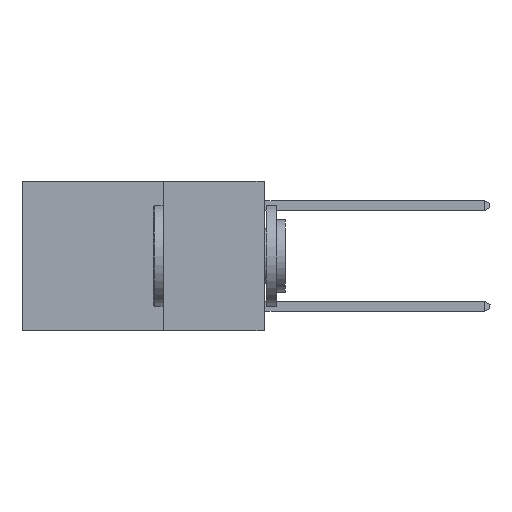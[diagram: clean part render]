
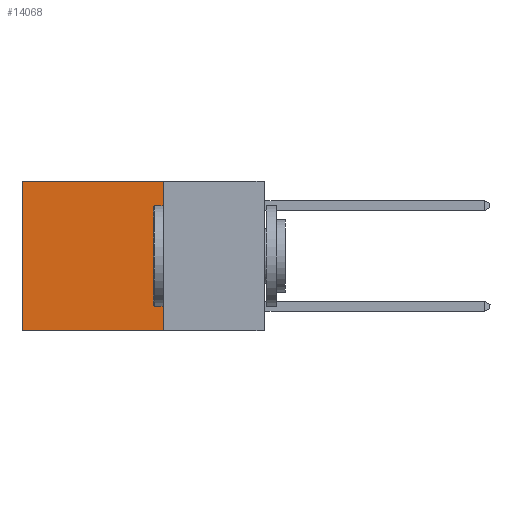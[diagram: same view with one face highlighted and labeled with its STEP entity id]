
A CAD part, left-side view. The second image highlights one B-rep face of the part: STEP entity #14068.
In plain terms, the highlighted planar face has unit normal (-1, 0, 0).
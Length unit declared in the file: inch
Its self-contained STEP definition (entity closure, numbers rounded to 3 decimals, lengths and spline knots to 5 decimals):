
#286 = CARTESIAN_POINT ( 'NONE',  ( 0.2625, 0.25, 0. ) ) ;
#1740 = AXIS2_PLACEMENT_3D ( 'NONE', #13962, #5261, #15449 ) ;
#1745 = EDGE_LOOP ( 'NONE', ( #13700, #10122, #11207, #15705 ) ) ;
#2292 = DIRECTION ( 'NONE',  ( 0., 0., -1. ) ) ;
#3195 = EDGE_CURVE ( 'NONE', #9516, #5290, #6839, .T. ) ;
#3809 = PLANE ( 'NONE',  #1740 ) ;
#4184 = EDGE_CURVE ( 'NONE', #5290, #18615, #13611, .T. ) ;
#5187 = EDGE_CURVE ( 'NONE', #9516, #7630, #16520, .T. ) ;
#5261 = DIRECTION ( 'NONE',  ( 1., 0., 0. ) ) ;
#5290 = VERTEX_POINT ( 'NONE', #10677 ) ;
#6839 = LINE ( 'NONE', #17581, #14090 ) ;
#7414 = DIRECTION ( 'NONE',  ( 0., 1., 0. ) ) ;
#7630 = VERTEX_POINT ( 'NONE', #16922 ) ;
#7952 = DIRECTION ( 'NONE',  ( 0., 1., 0. ) ) ;
#8009 = CARTESIAN_POINT ( 'NONE',  ( 0.2625, 0.25, 0. ) ) ;
#8986 = DIRECTION ( 'NONE',  ( 0., 0., -1. ) ) ;
#9244 = VECTOR ( 'NONE', #8986, 39.37008 ) ;
#9344 = CARTESIAN_POINT ( 'NONE',  ( 0.2625, 0.25, -0.37 ) ) ;
#9516 = VERTEX_POINT ( 'NONE', #8009 ) ;
#9976 = FACE_OUTER_BOUND ( 'NONE', #1745, .T. ) ;
#10122 = ORIENTED_EDGE ( 'NONE', *, *, #11447, .F. ) ;
#10677 = CARTESIAN_POINT ( 'NONE',  ( 0.2625, 0.6, 0. ) ) ;
#11207 = ORIENTED_EDGE ( 'NONE', *, *, #5187, .F. ) ;
#11447 = EDGE_CURVE ( 'NONE', #7630, #18615, #14175, .T. ) ;
#12444 = CARTESIAN_POINT ( 'NONE',  ( 0.2625, 0.6, 0. ) ) ;
#13151 = VECTOR ( 'NONE', #2292, 39.37008 ) ;
#13611 = LINE ( 'NONE', #12444, #13151 ) ;
#13700 = ORIENTED_EDGE ( 'NONE', *, *, #4184, .T. ) ;
#13717 = VECTOR ( 'NONE', #7952, 39.37008 ) ;
#13962 = CARTESIAN_POINT ( 'NONE',  ( 0.2625, 0.25, 0. ) ) ;
#14068 = ADVANCED_FACE ( 'NONE', ( #9976 ), #3809, .F. ) ;
#14090 = VECTOR ( 'NONE', #7414, 39.37008 ) ;
#14175 = LINE ( 'NONE', #9344, #13717 ) ;
#15449 = DIRECTION ( 'NONE',  ( 0., 0., -1. ) ) ;
#15705 = ORIENTED_EDGE ( 'NONE', *, *, #3195, .T. ) ;
#16520 = LINE ( 'NONE', #286, #9244 ) ;
#16922 = CARTESIAN_POINT ( 'NONE',  ( 0.2625, 0.25, -0.37 ) ) ;
#17581 = CARTESIAN_POINT ( 'NONE',  ( 0.2625, 0.25, 0. ) ) ;
#18615 = VERTEX_POINT ( 'NONE', #18740 ) ;
#18740 = CARTESIAN_POINT ( 'NONE',  ( 0.2625, 0.6, -0.37 ) ) ;
